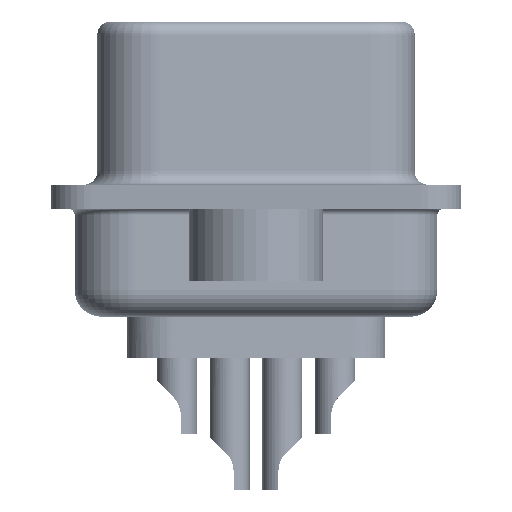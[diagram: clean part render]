
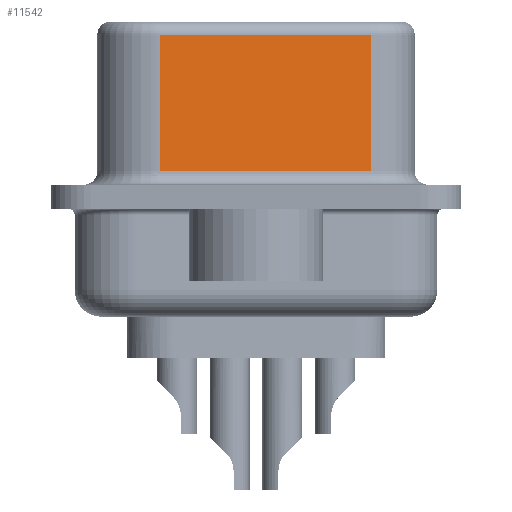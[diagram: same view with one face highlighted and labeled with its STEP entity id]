
A CAD part, left-side view. The second image highlights one B-rep face of the part: STEP entity #11542.
In plain terms, the highlighted planar face has unit normal (-0.985, -0.174, 0).
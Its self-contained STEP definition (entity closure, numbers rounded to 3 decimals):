
#496 = VECTOR ( 'NONE', #5626, 1000. ) ;
#2249 = VECTOR ( 'NONE', #34185, 1000. ) ;
#5626 = DIRECTION ( 'NONE',  ( 0., 0., -1. ) ) ;
#7282 = CARTESIAN_POINT ( 'NONE',  ( 3.735, 3.603, 0.95 ) ) ;
#7850 = CARTESIAN_POINT ( 'NONE',  ( 5.128, -4.297, 0.95 ) ) ;
#9824 = DIRECTION ( 'NONE',  ( -0.174, 0.985, 0. ) ) ;
#10000 = ORIENTED_EDGE ( 'NONE', *, *, #31909, .F. ) ;
#11542 = ADVANCED_FACE ( 'NONE', ( #40169 ), #33649, .F. ) ;
#14486 = CARTESIAN_POINT ( 'NONE',  ( 5.128, -4.297, 6.57 ) ) ;
#15357 = ORIENTED_EDGE ( 'NONE', *, *, #29144, .T. ) ;
#17214 = ORIENTED_EDGE ( 'NONE', *, *, #35434, .T. ) ;
#19090 = CARTESIAN_POINT ( 'NONE',  ( 5.128, -4.297, 6.07 ) ) ;
#20122 = DIRECTION ( 'NONE',  ( 0., 0., -1. ) ) ;
#21307 = LINE ( 'NONE', #7850, #2249 ) ;
#21966 = CARTESIAN_POINT ( 'NONE',  ( 5.128, -4.297, 6.07 ) ) ;
#22031 = LINE ( 'NONE', #34496, #496 ) ;
#23668 = VERTEX_POINT ( 'NONE', #37795 ) ;
#24841 = ORIENTED_EDGE ( 'NONE', *, *, #28459, .T. ) ;
#27837 = VECTOR ( 'NONE', #9824, 1000. ) ;
#28458 = AXIS2_PLACEMENT_3D ( 'NONE', #14486, #30885, #37429 ) ;
#28459 = EDGE_CURVE ( 'NONE', #31984, #31761, #21307, .T. ) ;
#28877 = EDGE_LOOP ( 'NONE', ( #10000, #15357, #17214, #24841 ) ) ;
#28964 = CARTESIAN_POINT ( 'NONE',  ( 5.128, -4.297, 6.57 ) ) ;
#29144 = EDGE_CURVE ( 'NONE', #30915, #23668, #34902, .T. ) ;
#30885 = DIRECTION ( 'NONE',  ( 0.985, 0.174, 0. ) ) ;
#30915 = VERTEX_POINT ( 'NONE', #21966 ) ;
#31761 = VERTEX_POINT ( 'NONE', #40246 ) ;
#31909 = EDGE_CURVE ( 'NONE', #30915, #31761, #38686, .T. ) ;
#31984 = VERTEX_POINT ( 'NONE', #7282 ) ;
#33649 = PLANE ( 'NONE',  #28458 ) ;
#34007 = VECTOR ( 'NONE', #20122, 1000. ) ;
#34185 = DIRECTION ( 'NONE',  ( 0.174, -0.985, 0. ) ) ;
#34496 = CARTESIAN_POINT ( 'NONE',  ( 3.735, 3.603, 6.57 ) ) ;
#34902 = LINE ( 'NONE', #19090, #27837 ) ;
#35434 = EDGE_CURVE ( 'NONE', #23668, #31984, #22031, .T. ) ;
#37429 = DIRECTION ( 'NONE',  ( -0.174, 0.985, 0. ) ) ;
#37795 = CARTESIAN_POINT ( 'NONE',  ( 3.735, 3.603, 6.07 ) ) ;
#38686 = LINE ( 'NONE', #28964, #34007 ) ;
#40169 = FACE_OUTER_BOUND ( 'NONE', #28877, .T. ) ;
#40246 = CARTESIAN_POINT ( 'NONE',  ( 5.128, -4.297, 0.95 ) ) ;
